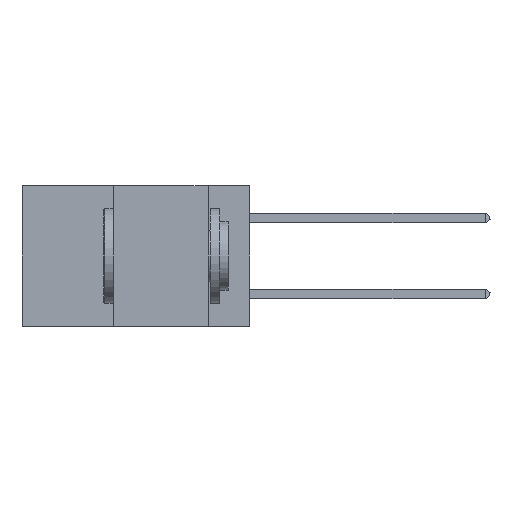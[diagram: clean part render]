
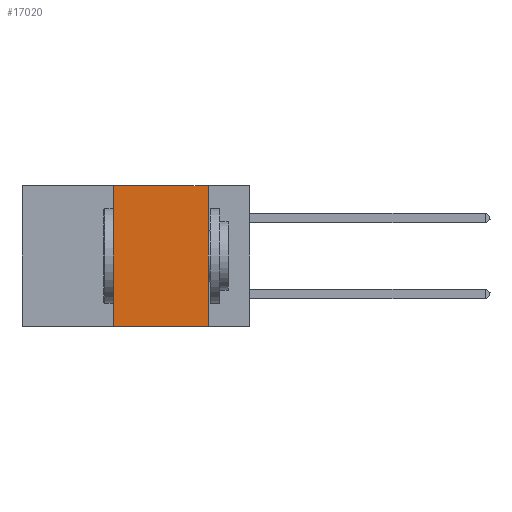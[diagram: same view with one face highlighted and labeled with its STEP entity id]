
A CAD part, left-side view. The second image highlights one B-rep face of the part: STEP entity #17020.
In plain terms, the highlighted planar face has unit normal (-1, 0, 0).
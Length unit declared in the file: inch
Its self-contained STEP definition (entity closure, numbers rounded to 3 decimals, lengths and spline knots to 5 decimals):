
#2074 = CARTESIAN_POINT ( 'NONE',  ( 0., 0.6, 0. ) ) ;
#2769 = CARTESIAN_POINT ( 'NONE',  ( 0., 0.6, 0. ) ) ;
#4485 = FACE_OUTER_BOUND ( 'NONE', #15502, .T. ) ;
#5914 = VERTEX_POINT ( 'NONE', #20437 ) ;
#5982 = ORIENTED_EDGE ( 'NONE', *, *, #9404, .F. ) ;
#7081 = VECTOR ( 'NONE', #31625, 39.37008 ) ;
#7396 = CARTESIAN_POINT ( 'NONE',  ( 0., 0.36, 0. ) ) ;
#9404 = EDGE_CURVE ( 'NONE', #30709, #32877, #24209, .T. ) ;
#10691 = VECTOR ( 'NONE', #36014, 39.37008 ) ;
#12060 = DIRECTION ( 'NONE',  ( 0., 0., -1. ) ) ;
#13817 = LINE ( 'NONE', #2769, #7081 ) ;
#15502 = EDGE_LOOP ( 'NONE', ( #5982, #23062, #33202, #26818 ) ) ;
#16282 = PLANE ( 'NONE',  #25984 ) ;
#17020 = ADVANCED_FACE ( 'NONE', ( #4485 ), #16282, .F. ) ;
#18142 = VERTEX_POINT ( 'NONE', #7396 ) ;
#18785 = CARTESIAN_POINT ( 'NONE',  ( 0., 0.36, 0. ) ) ;
#19867 = DIRECTION ( 'NONE',  ( 0., 0., -1. ) ) ;
#20437 = CARTESIAN_POINT ( 'NONE',  ( 0., 0.36, -0.37 ) ) ;
#20716 = CARTESIAN_POINT ( 'NONE',  ( 0., 0.6, -0.37 ) ) ;
#22017 = DIRECTION ( 'NONE',  ( 1., 0., 0. ) ) ;
#23062 = ORIENTED_EDGE ( 'NONE', *, *, #33482, .F. ) ;
#23487 = CARTESIAN_POINT ( 'NONE',  ( 0., 0.11, -0.37 ) ) ;
#23851 = EDGE_CURVE ( 'NONE', #5914, #32877, #32167, .T. ) ;
#24199 = DIRECTION ( 'NONE',  ( 0., 0., 1. ) ) ;
#24209 = LINE ( 'NONE', #31432, #35407 ) ;
#25984 = AXIS2_PLACEMENT_3D ( 'NONE', #2074, #22017, #12060 ) ;
#26000 = VECTOR ( 'NONE', #24199, 39.37008 ) ;
#26818 = ORIENTED_EDGE ( 'NONE', *, *, #23851, .T. ) ;
#28812 = CARTESIAN_POINT ( 'NONE',  ( 0., 0.11, 0. ) ) ;
#30709 = VERTEX_POINT ( 'NONE', #28812 ) ;
#31432 = CARTESIAN_POINT ( 'NONE',  ( 0., 0.11, 0. ) ) ;
#31625 = DIRECTION ( 'NONE',  ( 0., -1., 0. ) ) ;
#31725 = EDGE_CURVE ( 'NONE', #5914, #18142, #33630, .T. ) ;
#32167 = LINE ( 'NONE', #20716, #10691 ) ;
#32877 = VERTEX_POINT ( 'NONE', #23487 ) ;
#33202 = ORIENTED_EDGE ( 'NONE', *, *, #31725, .F. ) ;
#33482 = EDGE_CURVE ( 'NONE', #18142, #30709, #13817, .T. ) ;
#33630 = LINE ( 'NONE', #18785, #26000 ) ;
#35407 = VECTOR ( 'NONE', #19867, 39.37008 ) ;
#36014 = DIRECTION ( 'NONE',  ( 0., -1., 0. ) ) ;
